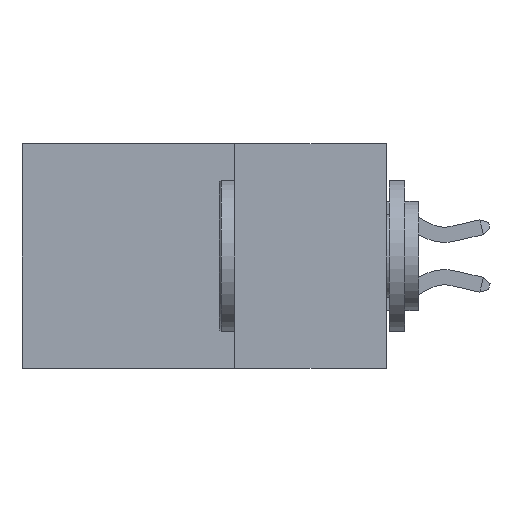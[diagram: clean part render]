
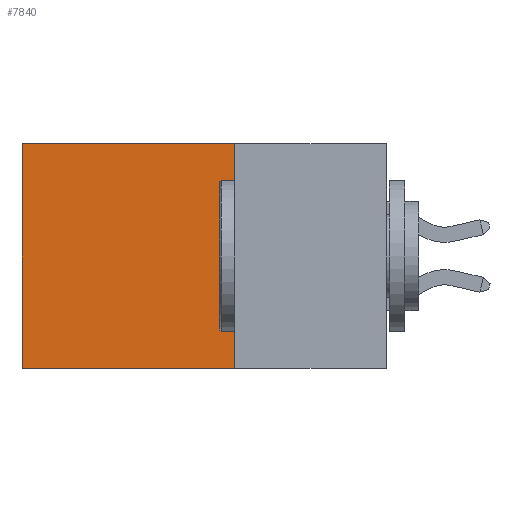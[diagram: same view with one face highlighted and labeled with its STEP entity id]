
A CAD part, left-side view. The second image highlights one B-rep face of the part: STEP entity #7840.
In plain terms, the highlighted planar face has unit normal (-1, 0, 0).
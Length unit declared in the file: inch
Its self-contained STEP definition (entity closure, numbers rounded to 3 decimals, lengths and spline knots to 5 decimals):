
#526 = LINE ( 'NONE', #13608, #9356 ) ;
#1182 = EDGE_LOOP ( 'NONE', ( #22655, #1726, #16323, #20051 ) ) ;
#1522 = DIRECTION ( 'NONE',  ( 0., 0., -1. ) ) ;
#1726 = ORIENTED_EDGE ( 'NONE', *, *, #8954, .F. ) ;
#2540 = EDGE_CURVE ( 'NONE', #6350, #20054, #11474, .T. ) ;
#4406 = DIRECTION ( 'NONE',  ( 0., 1., 0. ) ) ;
#4751 = VECTOR ( 'NONE', #4406, 39.37008 ) ;
#5304 = LINE ( 'NONE', #13195, #4751 ) ;
#5882 = LINE ( 'NONE', #19243, #14729 ) ;
#6240 = VECTOR ( 'NONE', #15081, 39.37008 ) ;
#6350 = VERTEX_POINT ( 'NONE', #13444 ) ;
#7840 = ADVANCED_FACE ( 'NONE', ( #9488 ), #15555, .F. ) ;
#8488 = CARTESIAN_POINT ( 'NONE',  ( 0.2615, 0.25, -0.37 ) ) ;
#8954 = EDGE_CURVE ( 'NONE', #10263, #20054, #5882, .T. ) ;
#9356 = VECTOR ( 'NONE', #21054, 39.37008 ) ;
#9488 = FACE_OUTER_BOUND ( 'NONE', #1182, .T. ) ;
#9925 = EDGE_CURVE ( 'NONE', #19195, #6350, #5304, .T. ) ;
#10263 = VERTEX_POINT ( 'NONE', #15810 ) ;
#11474 = LINE ( 'NONE', #15217, #6240 ) ;
#12062 = DIRECTION ( 'NONE',  ( 1., 0., 0. ) ) ;
#12528 = CARTESIAN_POINT ( 'NONE',  ( 0.2615, 0.6, -0.37 ) ) ;
#13195 = CARTESIAN_POINT ( 'NONE',  ( 0.2615, 0.25, 0. ) ) ;
#13444 = CARTESIAN_POINT ( 'NONE',  ( 0.2615, 0.6, 0. ) ) ;
#13608 = CARTESIAN_POINT ( 'NONE',  ( 0.2615, 0.25, -0.37 ) ) ;
#14729 = VECTOR ( 'NONE', #22707, 39.37008 ) ;
#15081 = DIRECTION ( 'NONE',  ( 0., 0., -1. ) ) ;
#15217 = CARTESIAN_POINT ( 'NONE',  ( 0.2615, 0.6, -0.37 ) ) ;
#15555 = PLANE ( 'NONE',  #21564 ) ;
#15810 = CARTESIAN_POINT ( 'NONE',  ( 0.2615, 0.25, -0.37 ) ) ;
#16323 = ORIENTED_EDGE ( 'NONE', *, *, #20828, .F. ) ;
#17190 = CARTESIAN_POINT ( 'NONE',  ( 0.2615, 0.25, 0. ) ) ;
#19195 = VERTEX_POINT ( 'NONE', #17190 ) ;
#19243 = CARTESIAN_POINT ( 'NONE',  ( 0.2615, 0.25, -0.37 ) ) ;
#20051 = ORIENTED_EDGE ( 'NONE', *, *, #9925, .T. ) ;
#20054 = VERTEX_POINT ( 'NONE', #12528 ) ;
#20828 = EDGE_CURVE ( 'NONE', #19195, #10263, #526, .T. ) ;
#21054 = DIRECTION ( 'NONE',  ( 0., 0., -1. ) ) ;
#21564 = AXIS2_PLACEMENT_3D ( 'NONE', #8488, #12062, #1522 ) ;
#22655 = ORIENTED_EDGE ( 'NONE', *, *, #2540, .T. ) ;
#22707 = DIRECTION ( 'NONE',  ( 0., 1., 0. ) ) ;
